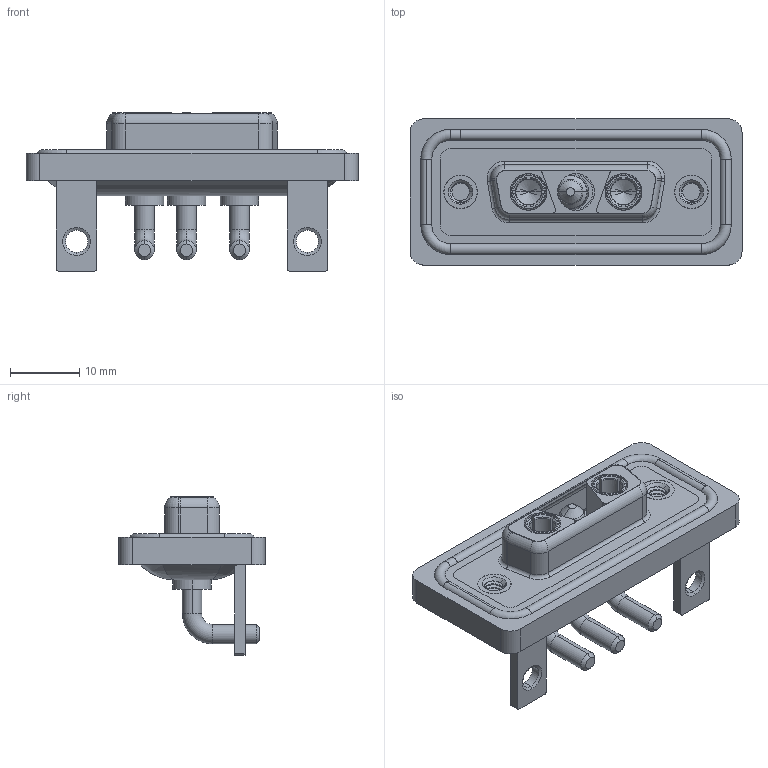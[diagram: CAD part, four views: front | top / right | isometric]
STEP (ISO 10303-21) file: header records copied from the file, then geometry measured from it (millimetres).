
FILE_DESCRIPTION (( 'STEP AP203' ), '1' );
FILE_NAME ('630W3WK3640-2NC.STEP', '2024-04-11T23:06:15', ( '' ), ( '' ), 'SwSTEP 2.0', 'SolidWorks 2023', '' );
FILE_SCHEMA (( 'CONFIG_CONTROL_DESIGN' ));
Length unit declared in the file: millimetre
Products named in the file (9): Power Socket_20A RA; 630Combo Shell Front_15 Contacts; 630Combo Housing_3WK3; 630W3WK3640-2NC; 630Combo Threaded Rivet_A; 630Combo Shell Rear_15 Contacts; Power Pin_20A RA; 630Combo Stabilizer Bracket_50 Contacts; 630Combo Waterproof Housing_15 Contacts
Assembly tree (11 placements, depth 2):
  630W3WK3640-2NC
    630Combo Housing_3WK3
    630Combo Shell Front_15 Contacts
    630Combo Shell Rear_15 Contacts
    630Combo Threaded Rivet_A  x2
    630Combo Stabilizer Bracket_50 Contacts  x2
    Power Socket_20A RA  x2
    Power Pin_20A RA
    630Combo Waterproof Housing_15 Contacts
Bounding box: 47.9 x 21.1 x 22.8 mm (x, y, z)
Volume: 6391.1 mm3; surface area: 10476.9 mm2
Topology: 15 solids, 15 shells, 637 faces, 1602 edges, 1014 vertices
Faces by surface type: cylinder 286, plane 198, torus 87, cone 53, bspline 13
Entity records: 18222 total; most frequent: CARTESIAN_POINT 4852, DIRECTION 2733, ORIENTED_EDGE 2520, EDGE_CURVE 1260, AXIS2_PLACEMENT_3D 1093, VERTEX_POINT 799, CIRCLE 578, EDGE_LOOP 563
